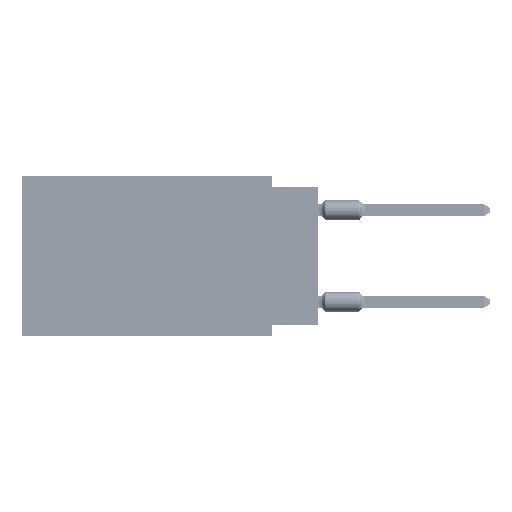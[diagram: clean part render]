
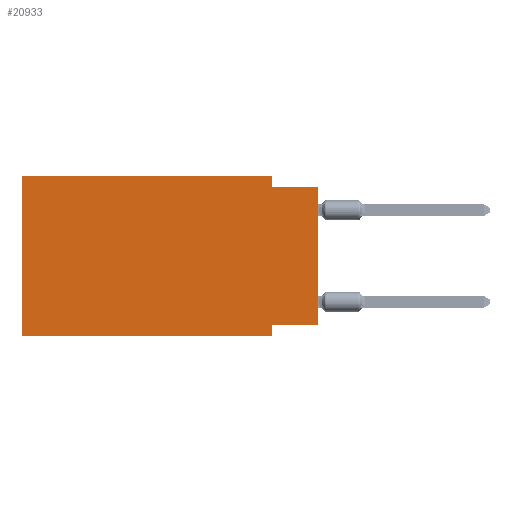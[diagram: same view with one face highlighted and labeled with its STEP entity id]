
A CAD part, left-side view. The second image highlights one B-rep face of the part: STEP entity #20933.
In plain terms, the highlighted planar face has unit normal (-1, 0, 0).
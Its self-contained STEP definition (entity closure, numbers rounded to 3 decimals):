
#2425 = ORIENTED_EDGE ( 'NONE', *, *, #63622, .F. ) ;
#2735 = DIRECTION ( 'NONE',  ( 0., -1., 0. ) ) ;
#3900 = VECTOR ( 'NONE', #13572, 1000. ) ;
#3988 = DIRECTION ( 'NONE',  ( 0., 0., 1. ) ) ;
#4365 = VERTEX_POINT ( 'NONE', #42638 ) ;
#4378 = LINE ( 'NONE', #22626, #61347 ) ;
#5423 = ORIENTED_EDGE ( 'NONE', *, *, #19819, .F. ) ;
#7310 = ORIENTED_EDGE ( 'NONE', *, *, #13814, .F. ) ;
#9684 = VERTEX_POINT ( 'NONE', #65389 ) ;
#9857 = LINE ( 'NONE', #45975, #60405 ) ;
#12355 = DIRECTION ( 'NONE',  ( 0., -1., 0. ) ) ;
#13572 = DIRECTION ( 'NONE',  ( 0., 0., -1. ) ) ;
#13814 = EDGE_CURVE ( 'NONE', #32790, #67138, #36596, .T. ) ;
#14736 = PLANE ( 'NONE',  #54957 ) ;
#15422 = EDGE_CURVE ( 'NONE', #4365, #72281, #26246, .T. ) ;
#17534 = CARTESIAN_POINT ( 'NONE',  ( 0., 2.54, -8.255 ) ) ;
#19582 = VECTOR ( 'NONE', #67088, 1000. ) ;
#19819 = EDGE_CURVE ( 'NONE', #9684, #33159, #4378, .T. ) ;
#20933 = ADVANCED_FACE ( 'NONE', ( #75449 ), #14736, .F. ) ;
#21082 = DIRECTION ( 'NONE',  ( 1., 0., 0. ) ) ;
#21383 = VECTOR ( 'NONE', #40830, 1000. ) ;
#22606 = ORIENTED_EDGE ( 'NONE', *, *, #43181, .F. ) ;
#22626 = CARTESIAN_POINT ( 'NONE',  ( 0., 16.383, 0. ) ) ;
#24311 = CARTESIAN_POINT ( 'NONE',  ( 0., 2.54, -8.89 ) ) ;
#26246 = LINE ( 'NONE', #38928, #58374 ) ;
#27931 = LINE ( 'NONE', #52123, #59059 ) ;
#28143 = CARTESIAN_POINT ( 'NONE',  ( 0., 2.54, 0. ) ) ;
#31283 = EDGE_CURVE ( 'NONE', #4365, #32790, #37854, .T. ) ;
#31623 = CARTESIAN_POINT ( 'NONE',  ( 0., 0., -0.635 ) ) ;
#32674 = EDGE_CURVE ( 'NONE', #37825, #72281, #43286, .T. ) ;
#32790 = VERTEX_POINT ( 'NONE', #17534 ) ;
#33159 = VERTEX_POINT ( 'NONE', #41254 ) ;
#36596 = LINE ( 'NONE', #54444, #3900 ) ;
#37825 = VERTEX_POINT ( 'NONE', #62192 ) ;
#37854 = LINE ( 'NONE', #42508, #19582 ) ;
#38483 = ORIENTED_EDGE ( 'NONE', *, *, #32674, .F. ) ;
#38928 = CARTESIAN_POINT ( 'NONE',  ( 0., 0., 0. ) ) ;
#39319 = DIRECTION ( 'NONE',  ( 0., 0., -1. ) ) ;
#39684 = ORIENTED_EDGE ( 'NONE', *, *, #52536, .T. ) ;
#40830 = DIRECTION ( 'NONE',  ( 0., 0., -1. ) ) ;
#41254 = CARTESIAN_POINT ( 'NONE',  ( 0., 16.383, 0. ) ) ;
#42132 = CARTESIAN_POINT ( 'NONE',  ( 0., 0., -0.635 ) ) ;
#42508 = CARTESIAN_POINT ( 'NONE',  ( 0., 0., -8.255 ) ) ;
#42638 = CARTESIAN_POINT ( 'NONE',  ( 0., 0., -8.255 ) ) ;
#43181 = EDGE_CURVE ( 'NONE', #55235, #37825, #70600, .T. ) ;
#43286 = LINE ( 'NONE', #42132, #48853 ) ;
#45975 = CARTESIAN_POINT ( 'NONE',  ( 0., 16.383, -8.89 ) ) ;
#48853 = VECTOR ( 'NONE', #12355, 1000. ) ;
#50834 = CARTESIAN_POINT ( 'NONE',  ( 0., 16.383, 0. ) ) ;
#51598 = DIRECTION ( 'NONE',  ( 0., 0., 1. ) ) ;
#52123 = CARTESIAN_POINT ( 'NONE',  ( 0., 16.383, 0. ) ) ;
#52245 = ORIENTED_EDGE ( 'NONE', *, *, #31283, .F. ) ;
#52536 = EDGE_CURVE ( 'NONE', #9684, #67138, #9857, .T. ) ;
#54444 = CARTESIAN_POINT ( 'NONE',  ( 0., 2.54, -8.89 ) ) ;
#54957 = AXIS2_PLACEMENT_3D ( 'NONE', #50834, #21082, #39319 ) ;
#55235 = VERTEX_POINT ( 'NONE', #28143 ) ;
#58374 = VECTOR ( 'NONE', #51598, 1000. ) ;
#58683 = CARTESIAN_POINT ( 'NONE',  ( 0., 2.54, 0. ) ) ;
#59059 = VECTOR ( 'NONE', #76355, 1000. ) ;
#60405 = VECTOR ( 'NONE', #2735, 1000. ) ;
#61347 = VECTOR ( 'NONE', #3988, 1000. ) ;
#62192 = CARTESIAN_POINT ( 'NONE',  ( 0., 2.54, -0.635 ) ) ;
#63622 = EDGE_CURVE ( 'NONE', #33159, #55235, #27931, .T. ) ;
#65389 = CARTESIAN_POINT ( 'NONE',  ( 0., 16.383, -8.89 ) ) ;
#65959 = ORIENTED_EDGE ( 'NONE', *, *, #15422, .T. ) ;
#67088 = DIRECTION ( 'NONE',  ( 0., 1., 0. ) ) ;
#67138 = VERTEX_POINT ( 'NONE', #24311 ) ;
#70600 = LINE ( 'NONE', #58683, #21383 ) ;
#72281 = VERTEX_POINT ( 'NONE', #31623 ) ;
#72873 = EDGE_LOOP ( 'NONE', ( #65959, #38483, #22606, #2425, #5423, #39684, #7310, #52245 ) ) ;
#75449 = FACE_OUTER_BOUND ( 'NONE', #72873, .T. ) ;
#76355 = DIRECTION ( 'NONE',  ( 0., -1., 0. ) ) ;
